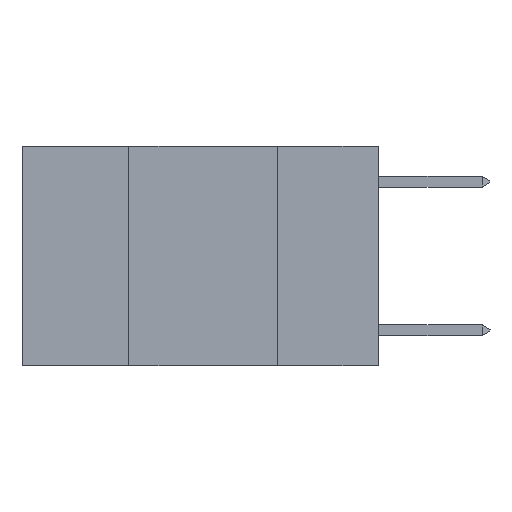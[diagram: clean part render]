
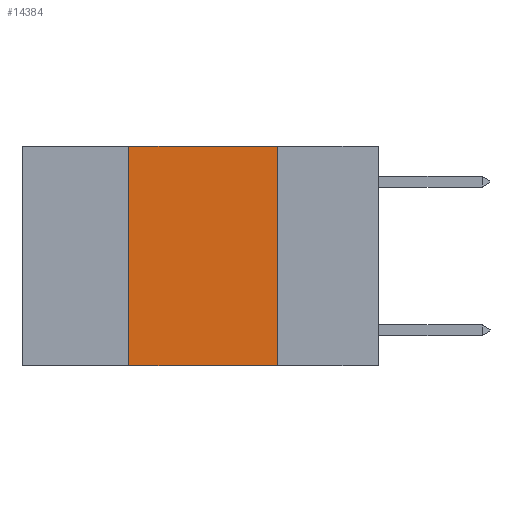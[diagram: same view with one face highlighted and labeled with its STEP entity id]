
A CAD part, left-side view. The second image highlights one B-rep face of the part: STEP entity #14384.
In plain terms, the highlighted planar face has unit normal (-1, 0, 0).
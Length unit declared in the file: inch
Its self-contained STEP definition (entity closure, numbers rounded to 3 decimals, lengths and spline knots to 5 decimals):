
#304 = CARTESIAN_POINT ( 'NONE',  ( 0., 0.42, -0.37 ) ) ;
#880 = ORIENTED_EDGE ( 'NONE', *, *, #10928, .T. ) ;
#1001 = ORIENTED_EDGE ( 'NONE', *, *, #13896, .F. ) ;
#1059 = ORIENTED_EDGE ( 'NONE', *, *, #19135, .F. ) ;
#1722 = ORIENTED_EDGE ( 'NONE', *, *, #11300, .F. ) ;
#2832 = VERTEX_POINT ( 'NONE', #9498 ) ;
#3522 = CARTESIAN_POINT ( 'NONE',  ( 0., 0.6, -0.37 ) ) ;
#3698 = VECTOR ( 'NONE', #18998, 39.37008 ) ;
#3857 = LINE ( 'NONE', #5034, #3698 ) ;
#4483 = DIRECTION ( 'NONE',  ( 0., 0., -1. ) ) ;
#5034 = CARTESIAN_POINT ( 'NONE',  ( 0., 0.6, 0. ) ) ;
#5298 = VERTEX_POINT ( 'NONE', #18837 ) ;
#6806 = DIRECTION ( 'NONE',  ( 0., -1., 0. ) ) ;
#6878 = VERTEX_POINT ( 'NONE', #14034 ) ;
#7798 = PLANE ( 'NONE',  #17815 ) ;
#8844 = FACE_OUTER_BOUND ( 'NONE', #10363, .T. ) ;
#9490 = DIRECTION ( 'NONE',  ( 0., 0., -1. ) ) ;
#9498 = CARTESIAN_POINT ( 'NONE',  ( 0., 0.17, -0.37 ) ) ;
#9722 = CARTESIAN_POINT ( 'NONE',  ( 0., 0.42, 0. ) ) ;
#10363 = EDGE_LOOP ( 'NONE', ( #1722, #1059, #1001, #880 ) ) ;
#10928 = EDGE_CURVE ( 'NONE', #19300, #2832, #19167, .T. ) ;
#11300 = EDGE_CURVE ( 'NONE', #6878, #2832, #16270, .T. ) ;
#11332 = DIRECTION ( 'NONE',  ( 0., 0., 1. ) ) ;
#12548 = CARTESIAN_POINT ( 'NONE',  ( 0., 0.6, 0. ) ) ;
#12584 = CARTESIAN_POINT ( 'NONE',  ( 0., 0.17, 0. ) ) ;
#13896 = EDGE_CURVE ( 'NONE', #19300, #5298, #14976, .T. ) ;
#14034 = CARTESIAN_POINT ( 'NONE',  ( 0., 0.17, 0. ) ) ;
#14384 = ADVANCED_FACE ( 'NONE', ( #8844 ), #7798, .F. ) ;
#14399 = VECTOR ( 'NONE', #11332, 39.37008 ) ;
#14976 = LINE ( 'NONE', #9722, #14399 ) ;
#16270 = LINE ( 'NONE', #12584, #16520 ) ;
#16520 = VECTOR ( 'NONE', #4483, 39.37008 ) ;
#17815 = AXIS2_PLACEMENT_3D ( 'NONE', #12548, #18533, #9490 ) ;
#18533 = DIRECTION ( 'NONE',  ( 1., 0., 0. ) ) ;
#18741 = VECTOR ( 'NONE', #6806, 39.37008 ) ;
#18837 = CARTESIAN_POINT ( 'NONE',  ( 0., 0.42, 0. ) ) ;
#18998 = DIRECTION ( 'NONE',  ( 0., -1., 0. ) ) ;
#19135 = EDGE_CURVE ( 'NONE', #5298, #6878, #3857, .T. ) ;
#19167 = LINE ( 'NONE', #3522, #18741 ) ;
#19300 = VERTEX_POINT ( 'NONE', #304 ) ;
